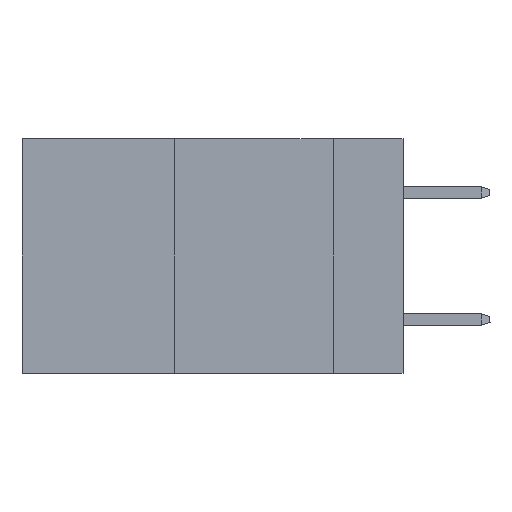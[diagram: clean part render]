
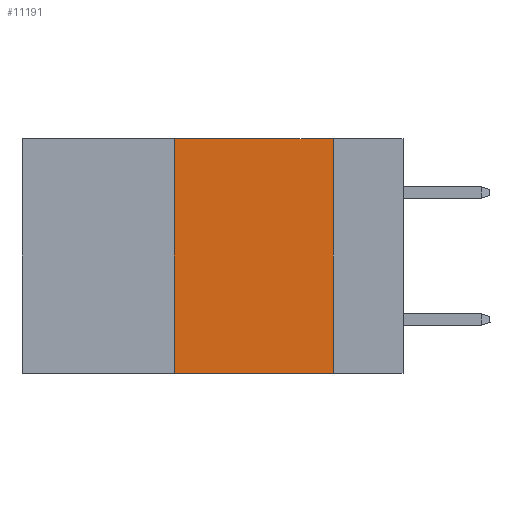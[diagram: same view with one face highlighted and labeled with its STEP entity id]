
A CAD part, left-side view. The second image highlights one B-rep face of the part: STEP entity #11191.
In plain terms, the highlighted planar face has unit normal (-1, 0, 0).
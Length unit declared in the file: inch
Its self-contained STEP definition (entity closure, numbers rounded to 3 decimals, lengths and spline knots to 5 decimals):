
#273 = LINE ( 'NONE', #3238, #7077 ) ;
#1643 = AXIS2_PLACEMENT_3D ( 'NONE', #5596, #2642, #4415 ) ;
#2162 = EDGE_CURVE ( 'NONE', #7339, #2345, #273, .T. ) ;
#2345 = VERTEX_POINT ( 'NONE', #11811 ) ;
#2499 = CARTESIAN_POINT ( 'NONE',  ( 0., 0.36, -0.37 ) ) ;
#2642 = DIRECTION ( 'NONE',  ( 1., 0., 0. ) ) ;
#2688 = CARTESIAN_POINT ( 'NONE',  ( 0., 0.36, 0. ) ) ;
#3007 = ORIENTED_EDGE ( 'NONE', *, *, #6333, .T. ) ;
#3122 = EDGE_CURVE ( 'NONE', #10773, #7339, #12345, .T. ) ;
#3238 = CARTESIAN_POINT ( 'NONE',  ( 0., 0.11, 0. ) ) ;
#3288 = CARTESIAN_POINT ( 'NONE',  ( 0., 0.36, 0. ) ) ;
#3351 = VECTOR ( 'NONE', #11786, 39.37008 ) ;
#4103 = LINE ( 'NONE', #9318, #11484 ) ;
#4209 = EDGE_CURVE ( 'NONE', #7146, #10773, #11716, .T. ) ;
#4415 = DIRECTION ( 'NONE',  ( 0., 0., -1. ) ) ;
#4745 = DIRECTION ( 'NONE',  ( 0., -1., 0. ) ) ;
#5596 = CARTESIAN_POINT ( 'NONE',  ( 0., 0.6, 0. ) ) ;
#6333 = EDGE_CURVE ( 'NONE', #7146, #2345, #4103, .T. ) ;
#7077 = VECTOR ( 'NONE', #8329, 39.37008 ) ;
#7146 = VERTEX_POINT ( 'NONE', #2499 ) ;
#7339 = VERTEX_POINT ( 'NONE', #11128 ) ;
#7849 = CARTESIAN_POINT ( 'NONE',  ( 0., 0.6, 0. ) ) ;
#8329 = DIRECTION ( 'NONE',  ( 0., 0., -1. ) ) ;
#9318 = CARTESIAN_POINT ( 'NONE',  ( 0., 0.6, -0.37 ) ) ;
#9355 = ORIENTED_EDGE ( 'NONE', *, *, #4209, .F. ) ;
#10602 = PLANE ( 'NONE',  #1643 ) ;
#10659 = VECTOR ( 'NONE', #4745, 39.37008 ) ;
#10773 = VERTEX_POINT ( 'NONE', #3288 ) ;
#11128 = CARTESIAN_POINT ( 'NONE',  ( 0., 0.11, 0. ) ) ;
#11191 = ADVANCED_FACE ( 'NONE', ( #12668 ), #10602, .F. ) ;
#11484 = VECTOR ( 'NONE', #12375, 39.37008 ) ;
#11716 = LINE ( 'NONE', #2688, #3351 ) ;
#11786 = DIRECTION ( 'NONE',  ( 0., 0., 1. ) ) ;
#11811 = CARTESIAN_POINT ( 'NONE',  ( 0., 0.11, -0.37 ) ) ;
#12345 = LINE ( 'NONE', #7849, #10659 ) ;
#12375 = DIRECTION ( 'NONE',  ( 0., -1., 0. ) ) ;
#12548 = ORIENTED_EDGE ( 'NONE', *, *, #2162, .F. ) ;
#12653 = ORIENTED_EDGE ( 'NONE', *, *, #3122, .F. ) ;
#12668 = FACE_OUTER_BOUND ( 'NONE', #12814, .T. ) ;
#12814 = EDGE_LOOP ( 'NONE', ( #12548, #12653, #9355, #3007 ) ) ;
